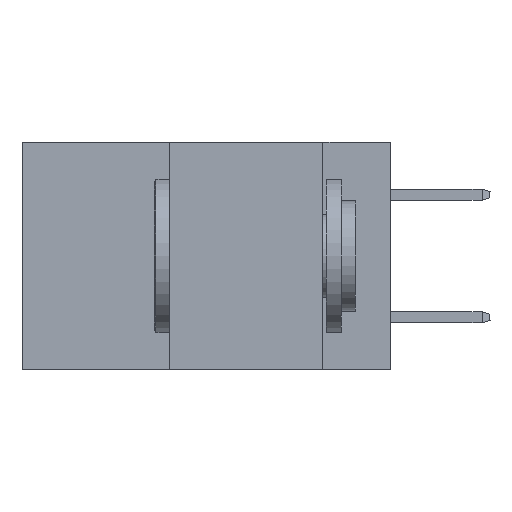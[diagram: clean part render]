
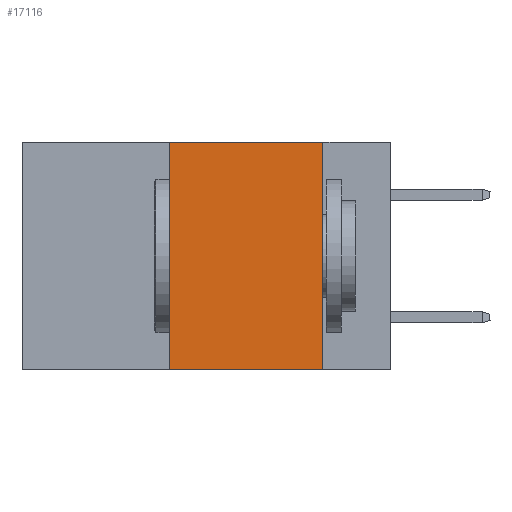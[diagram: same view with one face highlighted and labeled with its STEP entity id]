
A CAD part, left-side view. The second image highlights one B-rep face of the part: STEP entity #17116.
In plain terms, the highlighted planar face has unit normal (-1, 0, 0).
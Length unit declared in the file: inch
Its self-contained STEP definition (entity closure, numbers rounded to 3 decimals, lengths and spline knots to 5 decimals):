
#2672 = CARTESIAN_POINT ( 'NONE',  ( 0., 0.11, 0. ) ) ;
#3775 = DIRECTION ( 'NONE',  ( 0., 0., 1. ) ) ;
#3941 = PLANE ( 'NONE',  #37404 ) ;
#4561 = DIRECTION ( 'NONE',  ( 1., 0., 0. ) ) ;
#4732 = EDGE_CURVE ( 'NONE', #16738, #39525, #21240, .T. ) ;
#9868 = ORIENTED_EDGE ( 'NONE', *, *, #26521, .T. ) ;
#10042 = LINE ( 'NONE', #26024, #10598 ) ;
#10598 = VECTOR ( 'NONE', #11865, 39.37008 ) ;
#11865 = DIRECTION ( 'NONE',  ( 0., -1., 0. ) ) ;
#12182 = DIRECTION ( 'NONE',  ( 0., -1., 0. ) ) ;
#13866 = LINE ( 'NONE', #39641, #25580 ) ;
#14465 = VERTEX_POINT ( 'NONE', #38443 ) ;
#16738 = VERTEX_POINT ( 'NONE', #23496 ) ;
#17116 = ADVANCED_FACE ( 'NONE', ( #34622 ), #3941, .F. ) ;
#17194 = ORIENTED_EDGE ( 'NONE', *, *, #39001, .F. ) ;
#18291 = CARTESIAN_POINT ( 'NONE',  ( 0., 0.6, 0. ) ) ;
#21240 = LINE ( 'NONE', #2672, #29009 ) ;
#23496 = CARTESIAN_POINT ( 'NONE',  ( 0., 0.11, 0. ) ) ;
#24179 = ORIENTED_EDGE ( 'NONE', *, *, #4732, .F. ) ;
#24898 = VERTEX_POINT ( 'NONE', #41224 ) ;
#25495 = CARTESIAN_POINT ( 'NONE',  ( 0., 0.11, -0.37 ) ) ;
#25580 = VECTOR ( 'NONE', #3775, 39.37008 ) ;
#25626 = DIRECTION ( 'NONE',  ( 0., 0., -1. ) ) ;
#26024 = CARTESIAN_POINT ( 'NONE',  ( 0., 0.6, 0. ) ) ;
#26521 = EDGE_CURVE ( 'NONE', #14465, #39525, #41529, .T. ) ;
#26649 = CARTESIAN_POINT ( 'NONE',  ( 0., 0.6, -0.37 ) ) ;
#29009 = VECTOR ( 'NONE', #34939, 39.37008 ) ;
#31502 = EDGE_CURVE ( 'NONE', #14465, #24898, #13866, .T. ) ;
#32901 = EDGE_LOOP ( 'NONE', ( #24179, #17194, #38565, #9868 ) ) ;
#33673 = VECTOR ( 'NONE', #12182, 39.37008 ) ;
#34622 = FACE_OUTER_BOUND ( 'NONE', #32901, .T. ) ;
#34939 = DIRECTION ( 'NONE',  ( 0., 0., -1. ) ) ;
#37404 = AXIS2_PLACEMENT_3D ( 'NONE', #18291, #4561, #25626 ) ;
#38443 = CARTESIAN_POINT ( 'NONE',  ( 0., 0.36, -0.37 ) ) ;
#38565 = ORIENTED_EDGE ( 'NONE', *, *, #31502, .F. ) ;
#39001 = EDGE_CURVE ( 'NONE', #24898, #16738, #10042, .T. ) ;
#39525 = VERTEX_POINT ( 'NONE', #25495 ) ;
#39641 = CARTESIAN_POINT ( 'NONE',  ( 0., 0.36, 0. ) ) ;
#41224 = CARTESIAN_POINT ( 'NONE',  ( 0., 0.36, 0. ) ) ;
#41529 = LINE ( 'NONE', #26649, #33673 ) ;
